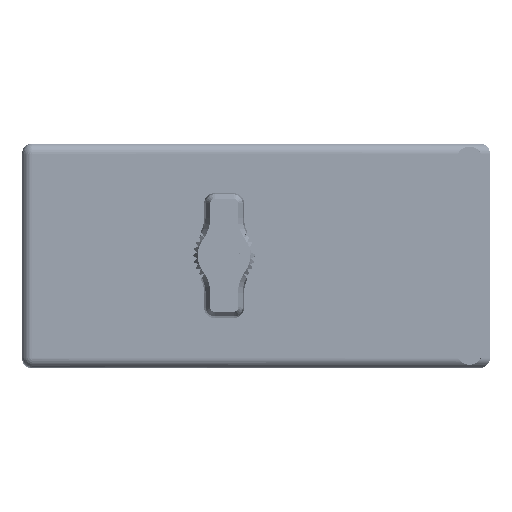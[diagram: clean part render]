
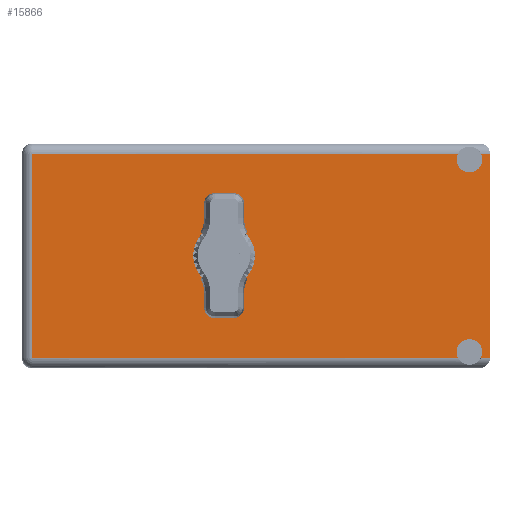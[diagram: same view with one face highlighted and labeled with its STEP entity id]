
A CAD part, top view. The second image highlights one B-rep face of the part: STEP entity #15866.
In plain terms, the highlighted face is planar.
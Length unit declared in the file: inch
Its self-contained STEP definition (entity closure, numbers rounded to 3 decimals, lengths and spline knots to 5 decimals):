
#1546 = CARTESIAN_POINT ( 'NONE',  ( 1.3775, 2.03, -0.765 ) ) ;
#3119 = EDGE_LOOP ( 'NONE', ( #10215, #5143, #52983, #33488, #33334, #107161, #35102, #9691, #6242, #69958 ) ) ;
#5143 = ORIENTED_EDGE ( 'NONE', *, *, #24980, .F. ) ;
#6020 = CARTESIAN_POINT ( 'NONE',  ( 0., 2.03, -1.53 ) ) ;
#6242 = ORIENTED_EDGE ( 'NONE', *, *, #16220, .T. ) ;
#6663 = DIRECTION ( 'NONE',  ( 0., 0., 1. ) ) ;
#7353 = AXIS2_PLACEMENT_3D ( 'NONE', #49607, #81684, #58094 ) ;
#8030 = VERTEX_POINT ( 'NONE', #101311 ) ;
#8046 = AXIS2_PLACEMENT_3D ( 'NONE', #1546, #25268, #33778 ) ;
#8205 = DIRECTION ( 'NONE',  ( -1., 0., 0. ) ) ;
#9691 = ORIENTED_EDGE ( 'NONE', *, *, #76202, .F. ) ;
#10215 = ORIENTED_EDGE ( 'NONE', *, *, #97172, .T. ) ;
#11131 = VERTEX_POINT ( 'NONE', #61624 ) ;
#12955 = CARTESIAN_POINT ( 'NONE',  ( 3.12833, 2.03, -1.46 ) ) ;
#13028 = CARTESIAN_POINT ( 'NONE',  ( 1.3775, 2.03, -0.935 ) ) ;
#14436 = AXIS2_PLACEMENT_3D ( 'NONE', #78678, #104460, #37386 ) ;
#14496 = CIRCLE ( 'NONE', #35086, 0.0875 ) ;
#15866 = ADVANCED_FACE ( 'NONE', ( #58535, #94164 ), #106338, .T. ) ;
#16220 = EDGE_CURVE ( 'NONE', #59538, #44916, #32091, .T. ) ;
#16300 = DIRECTION ( 'NONE',  ( 1., 0., 0. ) ) ;
#17044 = CIRCLE ( 'NONE', #39336, 0.0875 ) ;
#18763 = VECTOR ( 'NONE', #8205, 39.37008 ) ;
#24267 = VERTEX_POINT ( 'NONE', #31341 ) ;
#24980 = EDGE_CURVE ( 'NONE', #62887, #8030, #95445, .T. ) ;
#25268 = DIRECTION ( 'NONE',  ( 0., 1., 0. ) ) ;
#25466 = EDGE_CURVE ( 'NONE', #24267, #60178, #41303, .T. ) ;
#26694 = CARTESIAN_POINT ( 'NONE',  ( 3.05, 2.03, -0.109 ) ) ;
#29084 = AXIS2_PLACEMENT_3D ( 'NONE', #47702, #82320, #6663 ) ;
#29107 = VERTEX_POINT ( 'NONE', #83829 ) ;
#31341 = CARTESIAN_POINT ( 'NONE',  ( 3.05, 2.03, -1.3335 ) ) ;
#31804 = DIRECTION ( 'NONE',  ( 0., 0., 1. ) ) ;
#31807 = EDGE_CURVE ( 'NONE', #34899, #58647, #99470, .T. ) ;
#32091 = LINE ( 'NONE', #66900, #18763 ) ;
#33334 = ORIENTED_EDGE ( 'NONE', *, *, #49391, .F. ) ;
#33488 = ORIENTED_EDGE ( 'NONE', *, *, #31807, .T. ) ;
#33778 = DIRECTION ( 'NONE',  ( 0., 0., 1. ) ) ;
#34899 = VERTEX_POINT ( 'NONE', #86363 ) ;
#35086 = AXIS2_PLACEMENT_3D ( 'NONE', #26694, #85683, #94174 ) ;
#35102 = ORIENTED_EDGE ( 'NONE', *, *, #25466, .F. ) ;
#37386 = DIRECTION ( 'NONE',  ( 0., 0., 1. ) ) ;
#38648 = VERTEX_POINT ( 'NONE', #64396 ) ;
#39336 = AXIS2_PLACEMENT_3D ( 'NONE', #90444, #39953, #31804 ) ;
#39953 = DIRECTION ( 'NONE',  ( 0., 1., 0. ) ) ;
#40584 = CARTESIAN_POINT ( 'NONE',  ( 0.07, 2.03, -1.46 ) ) ;
#41303 = CIRCLE ( 'NONE', #14436, 0.0875 ) ;
#41619 = ORIENTED_EDGE ( 'NONE', *, *, #64243, .F. ) ;
#44916 = VERTEX_POINT ( 'NONE', #40584 ) ;
#45025 = CARTESIAN_POINT ( 'NONE',  ( 3.19, 2.03, 0. ) ) ;
#47702 = CARTESIAN_POINT ( 'NONE',  ( 1.3775, 2.03, -0.765 ) ) ;
#49391 = EDGE_CURVE ( 'NONE', #29107, #58647, #93750, .T. ) ;
#49607 = CARTESIAN_POINT ( 'NONE',  ( 3.05, 2.03, -0.109 ) ) ;
#50466 = CIRCLE ( 'NONE', #8046, 0.17 ) ;
#51561 = VECTOR ( 'NONE', #94498, 39.37008 ) ;
#52983 = ORIENTED_EDGE ( 'NONE', *, *, #75914, .F. ) ;
#53427 = CARTESIAN_POINT ( 'NONE',  ( 3.05, 2.03, -0.1965 ) ) ;
#54458 = CARTESIAN_POINT ( 'NONE',  ( 0., 2.03, -1.46 ) ) ;
#54473 = CARTESIAN_POINT ( 'NONE',  ( 2.97167, 2.03, -1.46 ) ) ;
#58094 = DIRECTION ( 'NONE',  ( 0., 0., 1. ) ) ;
#58535 = FACE_BOUND ( 'NONE', #72129, .T. ) ;
#58595 = VECTOR ( 'NONE', #80986, 39.37008 ) ;
#58647 = VERTEX_POINT ( 'NONE', #59609 ) ;
#59538 = VERTEX_POINT ( 'NONE', #54473 ) ;
#59609 = CARTESIAN_POINT ( 'NONE',  ( 3.19, 2.03, -0.07 ) ) ;
#60178 = VERTEX_POINT ( 'NONE', #12955 ) ;
#60555 = CARTESIAN_POINT ( 'NONE',  ( 3.19, 2.03, -0.07 ) ) ;
#61624 = CARTESIAN_POINT ( 'NONE',  ( 1.3775, 2.03, -0.595 ) ) ;
#62583 = CARTESIAN_POINT ( 'NONE',  ( 0.07, 2.03, -1.53 ) ) ;
#62887 = VERTEX_POINT ( 'NONE', #53427 ) ;
#63636 = DIRECTION ( 'NONE',  ( 0., 1., 0. ) ) ;
#64243 = EDGE_CURVE ( 'NONE', #11131, #96798, #96858, .T. ) ;
#64396 = CARTESIAN_POINT ( 'NONE',  ( 0.07, 2.03, -0.07 ) ) ;
#66900 = CARTESIAN_POINT ( 'NONE',  ( 0., 2.03, -1.46 ) ) ;
#69958 = ORIENTED_EDGE ( 'NONE', *, *, #81762, .T. ) ;
#72129 = EDGE_LOOP ( 'NONE', ( #41619, #105376 ) ) ;
#75914 = EDGE_CURVE ( 'NONE', #34899, #62887, #14496, .T. ) ;
#76202 = EDGE_CURVE ( 'NONE', #59538, #24267, #17044, .T. ) ;
#77180 = EDGE_CURVE ( 'NONE', #29107, #60178, #89657, .T. ) ;
#78678 = CARTESIAN_POINT ( 'NONE',  ( 3.05, 2.03, -1.421 ) ) ;
#80280 = DIRECTION ( 'NONE',  ( -1., 0., 0. ) ) ;
#80986 = DIRECTION ( 'NONE',  ( 0., 0., 1. ) ) ;
#80990 = VECTOR ( 'NONE', #16300, 39.37008 ) ;
#81684 = DIRECTION ( 'NONE',  ( 0., 1., 0. ) ) ;
#81762 = EDGE_CURVE ( 'NONE', #44916, #38648, #98130, .T. ) ;
#82320 = DIRECTION ( 'NONE',  ( 0., 1., 0. ) ) ;
#82417 = CARTESIAN_POINT ( 'NONE',  ( 3.19, 2.03, -0.07 ) ) ;
#83829 = CARTESIAN_POINT ( 'NONE',  ( 3.19, 2.03, -1.46 ) ) ;
#83866 = EDGE_CURVE ( 'NONE', #96798, #11131, #50466, .T. ) ;
#85683 = DIRECTION ( 'NONE',  ( 0., 1., 0. ) ) ;
#86363 = CARTESIAN_POINT ( 'NONE',  ( 3.12833, 2.03, -0.07 ) ) ;
#87382 = LINE ( 'NONE', #60555, #51561 ) ;
#89657 = LINE ( 'NONE', #54458, #91030 ) ;
#90444 = CARTESIAN_POINT ( 'NONE',  ( 3.05, 2.03, -1.421 ) ) ;
#91030 = VECTOR ( 'NONE', #80280, 39.37008 ) ;
#91141 = VECTOR ( 'NONE', #103962, 39.37008 ) ;
#93750 = LINE ( 'NONE', #45025, #91141 ) ;
#94164 = FACE_OUTER_BOUND ( 'NONE', #3119, .T. ) ;
#94174 = DIRECTION ( 'NONE',  ( 0., 0., 1. ) ) ;
#94498 = DIRECTION ( 'NONE',  ( 1., 0., 0. ) ) ;
#95445 = CIRCLE ( 'NONE', #7353, 0.0875 ) ;
#96798 = VERTEX_POINT ( 'NONE', #13028 ) ;
#96858 = CIRCLE ( 'NONE', #29084, 0.17 ) ;
#97172 = EDGE_CURVE ( 'NONE', #38648, #8030, #87382, .T. ) ;
#98130 = LINE ( 'NONE', #62583, #58595 ) ;
#99470 = LINE ( 'NONE', #82417, #80990 ) ;
#101311 = CARTESIAN_POINT ( 'NONE',  ( 2.97167, 2.03, -0.07 ) ) ;
#101384 = AXIS2_PLACEMENT_3D ( 'NONE', #6020, #63636, #105978 ) ;
#103962 = DIRECTION ( 'NONE',  ( 0., 0., 1. ) ) ;
#104460 = DIRECTION ( 'NONE',  ( 0., 1., 0. ) ) ;
#105376 = ORIENTED_EDGE ( 'NONE', *, *, #83866, .F. ) ;
#105978 = DIRECTION ( 'NONE',  ( 0., 0., 1. ) ) ;
#106338 = PLANE ( 'NONE',  #101384 ) ;
#107161 = ORIENTED_EDGE ( 'NONE', *, *, #77180, .T. ) ;
